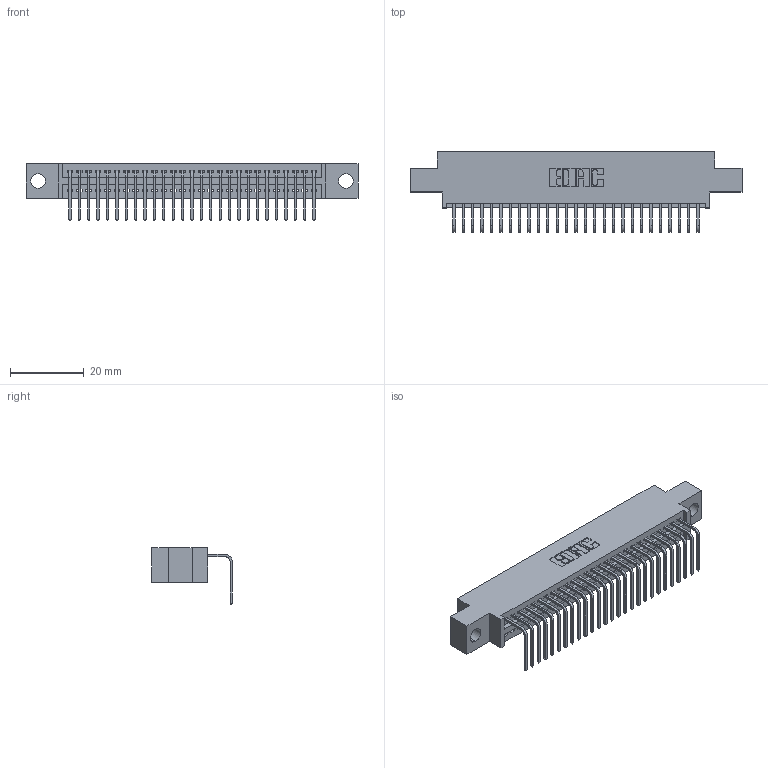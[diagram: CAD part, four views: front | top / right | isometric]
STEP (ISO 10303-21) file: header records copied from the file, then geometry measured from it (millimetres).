
FILE_DESCRIPTION (( 'STEP AP203' ), '1' );
FILE_NAME ('345-027-558-604.STEP', '2021-06-09T16:20:55', ( '' ), ( '' ), 'SwSTEP 2.0', 'SolidWorks 2020', '' );
FILE_SCHEMA (( 'CONFIG_CONTROL_DESIGN' ));
Length unit declared in the file: inch
Products named in the file (3): 345-027-558-604; 345 Part_0.170 Offset - 0.156 Dia-TI; 345-292-001_558 Tail - 2
Assembly tree (28 placements, depth 2):
  345-027-558-604
    345 Part_0.170 Offset - 0.156 Dia-TI
    345-292-001_558 Tail - 2  x27
Bounding box: 89.79 x 21.83 x 15.37 mm (x, y, z)
Volume: 8276 mm3; surface area: 11291.8 mm2
Topology: 28 solids, 28 shells, 1764 faces, 5303 edges, 3498 vertices
Faces by surface type: plane 1232, cylinder 532
Entity records: 22975 total; most frequent: CARTESIAN_POINT 3991, ORIENTED_EDGE 3950, DIRECTION 3505, EDGE_CURVE 1975, VECTOR 1735, LINE 1735, VERTEX_POINT 1314, AXIS2_PLACEMENT_3D 885
